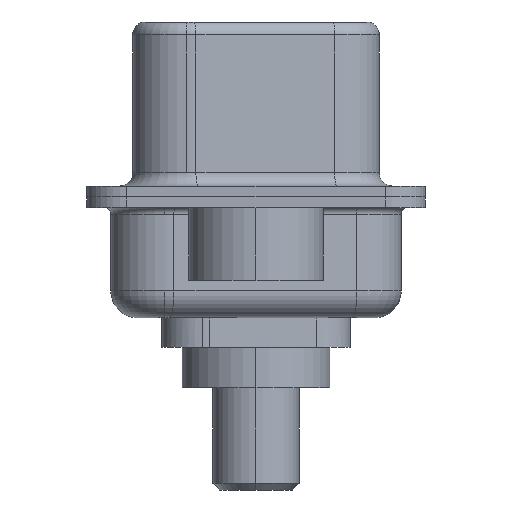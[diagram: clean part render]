
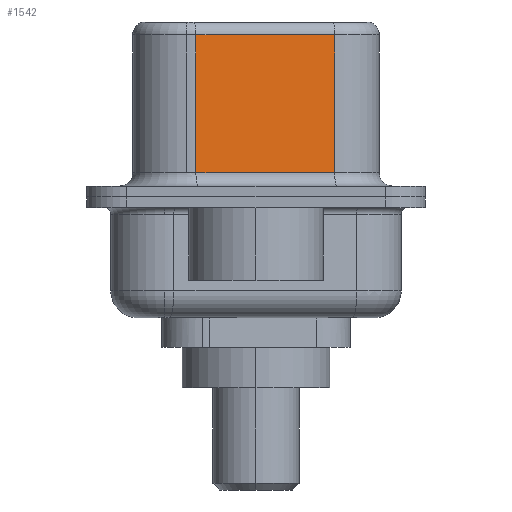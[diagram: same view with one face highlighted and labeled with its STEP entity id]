
A CAD part, left-side view. The second image highlights one B-rep face of the part: STEP entity #1542.
In plain terms, the highlighted planar face has unit normal (-0.985, -0.174, 0).
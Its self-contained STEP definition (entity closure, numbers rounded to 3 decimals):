
#3 = PLANE ( 'NONE',  #1587 ) ;
#390 = CARTESIAN_POINT ( 'NONE',  ( 3.655, 2.233, 6.02 ) ) ;
#1090 = VERTEX_POINT ( 'NONE', #12557 ) ;
#1542 = ADVANCED_FACE ( 'NONE', ( #6267 ), #3, .F. ) ;
#1562 = VERTEX_POINT ( 'NONE', #390 ) ;
#1576 = DIRECTION ( 'NONE',  ( -0.174, 0.985, 0. ) ) ;
#1587 = AXIS2_PLACEMENT_3D ( 'NONE', #2598, #2558, #1576 ) ;
#2368 = DIRECTION ( 'NONE',  ( 0., 0., -1. ) ) ;
#2558 = DIRECTION ( 'NONE',  ( 0.985, 0.174, 0. ) ) ;
#2598 = CARTESIAN_POINT ( 'NONE',  ( 4.565, -2.927, 6.52 ) ) ;
#2846 = CARTESIAN_POINT ( 'NONE',  ( 4.565, -2.927, 6.52 ) ) ;
#3010 = LINE ( 'NONE', #9604, #9042 ) ;
#3590 = VECTOR ( 'NONE', #3607, 1000. ) ;
#3607 = DIRECTION ( 'NONE',  ( 0.174, -0.985, 0. ) ) ;
#3654 = CARTESIAN_POINT ( 'NONE',  ( 3.655, 2.233, 0.9 ) ) ;
#4441 = ORIENTED_EDGE ( 'NONE', *, *, #12291, .T. ) ;
#4489 = CARTESIAN_POINT ( 'NONE',  ( 4.565, -2.927, 6.02 ) ) ;
#5579 = VECTOR ( 'NONE', #11259, 1000. ) ;
#6267 = FACE_OUTER_BOUND ( 'NONE', #15121, .T. ) ;
#6751 = LINE ( 'NONE', #10828, #3590 ) ;
#6870 = DIRECTION ( 'NONE',  ( -0.174, 0.985, 0. ) ) ;
#6915 = VERTEX_POINT ( 'NONE', #13998 ) ;
#8150 = ORIENTED_EDGE ( 'NONE', *, *, #13947, .T. ) ;
#8281 = LINE ( 'NONE', #4489, #11127 ) ;
#9042 = VECTOR ( 'NONE', #2368, 1000. ) ;
#9604 = CARTESIAN_POINT ( 'NONE',  ( 3.655, 2.233, 6.52 ) ) ;
#10828 = CARTESIAN_POINT ( 'NONE',  ( 4.565, -2.927, 0.9 ) ) ;
#11127 = VECTOR ( 'NONE', #6870, 1000. ) ;
#11259 = DIRECTION ( 'NONE',  ( 0., 0., -1. ) ) ;
#12164 = EDGE_CURVE ( 'NONE', #1090, #1562, #8281, .T. ) ;
#12291 = EDGE_CURVE ( 'NONE', #12339, #6915, #6751, .T. ) ;
#12339 = VERTEX_POINT ( 'NONE', #3654 ) ;
#12557 = CARTESIAN_POINT ( 'NONE',  ( 4.565, -2.927, 6.02 ) ) ;
#13832 = ORIENTED_EDGE ( 'NONE', *, *, #12164, .T. ) ;
#13947 = EDGE_CURVE ( 'NONE', #1562, #12339, #3010, .T. ) ;
#13998 = CARTESIAN_POINT ( 'NONE',  ( 4.565, -2.927, 0.9 ) ) ;
#14820 = EDGE_CURVE ( 'NONE', #1090, #6915, #15519, .T. ) ;
#15121 = EDGE_LOOP ( 'NONE', ( #15264, #13832, #8150, #4441 ) ) ;
#15264 = ORIENTED_EDGE ( 'NONE', *, *, #14820, .F. ) ;
#15519 = LINE ( 'NONE', #2846, #5579 ) ;
